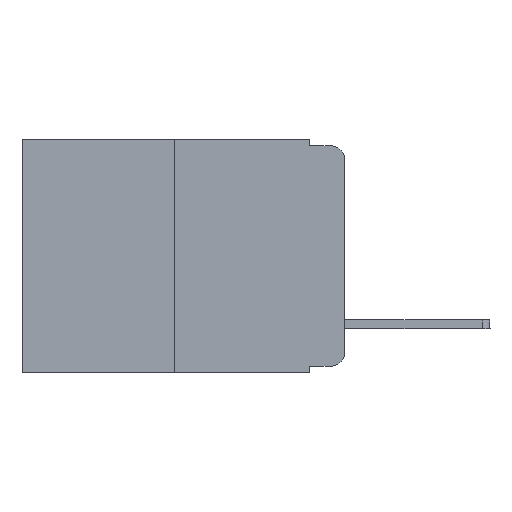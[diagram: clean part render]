
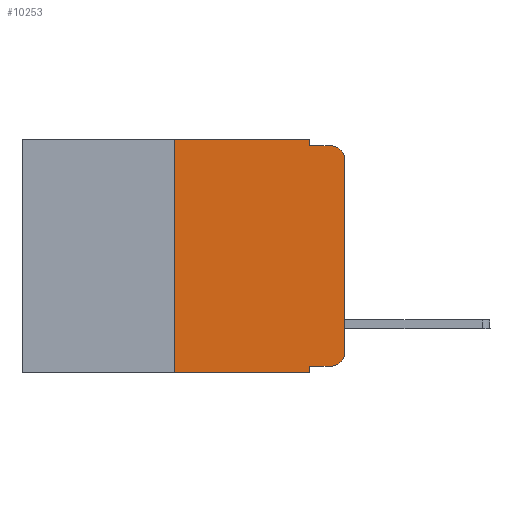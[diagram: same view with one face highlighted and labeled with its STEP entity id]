
A CAD part, left-side view. The second image highlights one B-rep face of the part: STEP entity #10253.
In plain terms, the highlighted planar face has unit normal (-1, 0, 0).
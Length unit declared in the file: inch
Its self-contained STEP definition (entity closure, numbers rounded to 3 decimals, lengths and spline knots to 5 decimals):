
#726 = EDGE_CURVE ( 'NONE', #9188, #7633, #13859, .T. ) ;
#1629 = VERTEX_POINT ( 'NONE', #7377 ) ;
#2344 = CARTESIAN_POINT ( 'NONE',  ( 0., 0.25, 0. ) ) ;
#2415 = CARTESIAN_POINT ( 'NONE',  ( 0., 0., 0. ) ) ;
#3019 = DIRECTION ( 'NONE',  ( 0., -1., 0. ) ) ;
#3033 = VERTEX_POINT ( 'NONE', #16988 ) ;
#3051 = EDGE_CURVE ( 'NONE', #8702, #1629, #13382, .T. ) ;
#3204 = EDGE_CURVE ( 'NONE', #3720, #8702, #11920, .T. ) ;
#3417 = EDGE_CURVE ( 'NONE', #6519, #16778, #5492, .T. ) ;
#3707 = LINE ( 'NONE', #4627, #4644 ) ;
#3720 = VERTEX_POINT ( 'NONE', #18501 ) ;
#4009 = CARTESIAN_POINT ( 'NONE',  ( 0., 0.25, -0.343 ) ) ;
#4627 = CARTESIAN_POINT ( 'NONE',  ( 0., 0.051, -0.333 ) ) ;
#4644 = VECTOR ( 'NONE', #3019, 39.37008 ) ;
#4650 = DIRECTION ( 'NONE',  ( 0., 0., 1. ) ) ;
#4887 = CARTESIAN_POINT ( 'NONE',  ( 0., 0.051, -0.01 ) ) ;
#5016 = EDGE_CURVE ( 'NONE', #16778, #1629, #16878, .T. ) ;
#5072 = VECTOR ( 'NONE', #18438, 39.37008 ) ;
#5469 = DIRECTION ( 'NONE',  ( -1., 0., 0. ) ) ;
#5492 = LINE ( 'NONE', #2415, #19406 ) ;
#5593 = CARTESIAN_POINT ( 'NONE',  ( 0., 0.02, -0.03 ) ) ;
#5607 = CARTESIAN_POINT ( 'NONE',  ( 0., 0., -0.03 ) ) ;
#5933 = EDGE_CURVE ( 'NONE', #3033, #6099, #3707, .T. ) ;
#6099 = VERTEX_POINT ( 'NONE', #17000 ) ;
#6436 = CARTESIAN_POINT ( 'NONE',  ( 0., 0.051, -0.343 ) ) ;
#6439 = EDGE_CURVE ( 'NONE', #3033, #7633, #13006, .T. ) ;
#6473 = EDGE_CURVE ( 'NONE', #6099, #6519, #10121, .T. ) ;
#6489 = DIRECTION ( 'NONE',  ( 0., -1., 0. ) ) ;
#6519 = VERTEX_POINT ( 'NONE', #13787 ) ;
#7377 = CARTESIAN_POINT ( 'NONE',  ( 0., 0.02, -0.01 ) ) ;
#7517 = ORIENTED_EDGE ( 'NONE', *, *, #3417, .T. ) ;
#7633 = VERTEX_POINT ( 'NONE', #6436 ) ;
#7670 = LINE ( 'NONE', #2344, #5072 ) ;
#8132 = VECTOR ( 'NONE', #6489, 39.37008 ) ;
#8282 = CARTESIAN_POINT ( 'NONE',  ( 0., 0.051, 0. ) ) ;
#8307 = AXIS2_PLACEMENT_3D ( 'NONE', #12616, #18603, #12680 ) ;
#8633 = ORIENTED_EDGE ( 'NONE', *, *, #5016, .T. ) ;
#8702 = VERTEX_POINT ( 'NONE', #16035 ) ;
#8964 = AXIS2_PLACEMENT_3D ( 'NONE', #15910, #15981, #13011 ) ;
#9185 = DIRECTION ( 'NONE',  ( 0., -1., 0. ) ) ;
#9188 = VERTEX_POINT ( 'NONE', #4009 ) ;
#9403 = EDGE_CURVE ( 'NONE', #9188, #16193, #7670, .T. ) ;
#9405 = PLANE ( 'NONE',  #8307 ) ;
#9429 = ORIENTED_EDGE ( 'NONE', *, *, #6439, .F. ) ;
#9616 = EDGE_LOOP ( 'NONE', ( #7517, #8633, #19285, #9935, #16603, #12060, #15255, #9429, #11588, #14080 ) ) ;
#9935 = ORIENTED_EDGE ( 'NONE', *, *, #3204, .F. ) ;
#10121 = CIRCLE ( 'NONE', #8964, 0.02 ) ;
#10253 = ADVANCED_FACE ( 'NONE', ( #11228 ), #9405, .F. ) ;
#11228 = FACE_OUTER_BOUND ( 'NONE', #9616, .T. ) ;
#11588 = ORIENTED_EDGE ( 'NONE', *, *, #5933, .T. ) ;
#11920 = LINE ( 'NONE', #17342, #16496 ) ;
#12060 = ORIENTED_EDGE ( 'NONE', *, *, #9403, .F. ) ;
#12256 = VECTOR ( 'NONE', #17385, 39.37008 ) ;
#12616 = CARTESIAN_POINT ( 'NONE',  ( 0., 0.473, 0. ) ) ;
#12680 = DIRECTION ( 'NONE',  ( 0., 0., -1. ) ) ;
#13006 = LINE ( 'NONE', #8282, #12256 ) ;
#13011 = DIRECTION ( 'NONE',  ( 0., 0., -1. ) ) ;
#13160 = EDGE_CURVE ( 'NONE', #16193, #3720, #16614, .T. ) ;
#13382 = LINE ( 'NONE', #4887, #8132 ) ;
#13787 = CARTESIAN_POINT ( 'NONE',  ( 0., 0., -0.313 ) ) ;
#13815 = CARTESIAN_POINT ( 'NONE',  ( 0., 0.473, 0. ) ) ;
#13819 = CARTESIAN_POINT ( 'NONE',  ( 0., 0.473, -0.343 ) ) ;
#13859 = LINE ( 'NONE', #13819, #14832 ) ;
#14080 = ORIENTED_EDGE ( 'NONE', *, *, #6473, .T. ) ;
#14832 = VECTOR ( 'NONE', #16836, 39.37008 ) ;
#15255 = ORIENTED_EDGE ( 'NONE', *, *, #726, .T. ) ;
#15910 = CARTESIAN_POINT ( 'NONE',  ( 0., 0.02, -0.313 ) ) ;
#15981 = DIRECTION ( 'NONE',  ( -1., 0., 0. ) ) ;
#16035 = CARTESIAN_POINT ( 'NONE',  ( 0., 0.051, -0.01 ) ) ;
#16193 = VERTEX_POINT ( 'NONE', #17184 ) ;
#16292 = DIRECTION ( 'NONE',  ( 0., 0., -1. ) ) ;
#16496 = VECTOR ( 'NONE', #18957, 39.37008 ) ;
#16603 = ORIENTED_EDGE ( 'NONE', *, *, #13160, .F. ) ;
#16614 = LINE ( 'NONE', #13815, #18784 ) ;
#16778 = VERTEX_POINT ( 'NONE', #5607 ) ;
#16836 = DIRECTION ( 'NONE',  ( 0., -1., 0. ) ) ;
#16878 = CIRCLE ( 'NONE', #17975, 0.02 ) ;
#16988 = CARTESIAN_POINT ( 'NONE',  ( 0., 0.051, -0.333 ) ) ;
#17000 = CARTESIAN_POINT ( 'NONE',  ( 0., 0.02, -0.333 ) ) ;
#17184 = CARTESIAN_POINT ( 'NONE',  ( 0., 0.25, 0. ) ) ;
#17342 = CARTESIAN_POINT ( 'NONE',  ( 0., 0.051, 0. ) ) ;
#17385 = DIRECTION ( 'NONE',  ( 0., 0., -1. ) ) ;
#17975 = AXIS2_PLACEMENT_3D ( 'NONE', #5593, #5469, #16292 ) ;
#18438 = DIRECTION ( 'NONE',  ( 0., 0., 1. ) ) ;
#18501 = CARTESIAN_POINT ( 'NONE',  ( 0., 0.051, 0. ) ) ;
#18603 = DIRECTION ( 'NONE',  ( 1., 0., 0. ) ) ;
#18784 = VECTOR ( 'NONE', #9185, 39.37008 ) ;
#18957 = DIRECTION ( 'NONE',  ( 0., 0., -1. ) ) ;
#19285 = ORIENTED_EDGE ( 'NONE', *, *, #3051, .F. ) ;
#19406 = VECTOR ( 'NONE', #4650, 39.37008 ) ;
